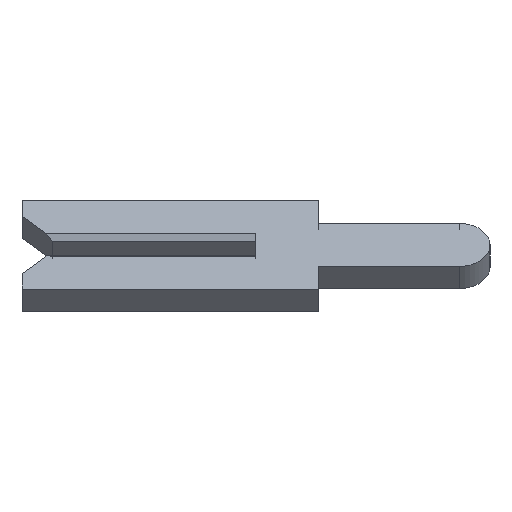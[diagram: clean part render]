
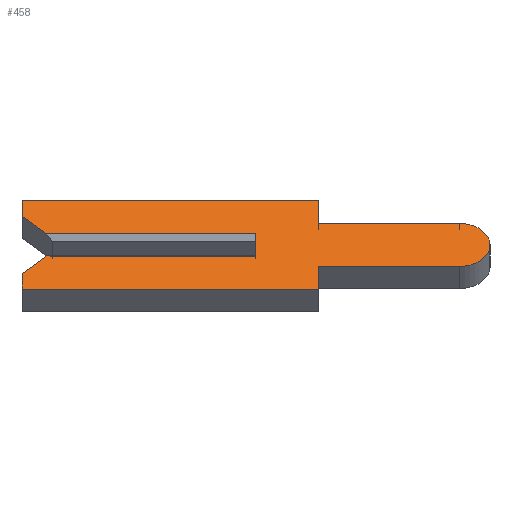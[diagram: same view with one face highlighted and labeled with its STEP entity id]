
A CAD part, left-side view. The second image highlights one B-rep face of the part: STEP entity #458.
In plain terms, the highlighted face is planar.
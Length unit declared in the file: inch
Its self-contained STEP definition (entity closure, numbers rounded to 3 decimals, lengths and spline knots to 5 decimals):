
#2 = LINE ( 'NONE', #1080, #922 ) ;
#7 = DIRECTION ( 'NONE',  ( 1., 0., 0. ) ) ;
#23 = VECTOR ( 'NONE', #225, 39.37008 ) ;
#26 = EDGE_CURVE ( 'NONE', #195, #709, #1039, .T. ) ;
#31 = CARTESIAN_POINT ( 'NONE',  ( -0.01, 0.15, -0.026 ) ) ;
#93 = DIRECTION ( 'NONE',  ( 0., 0., 1. ) ) ;
#110 = CARTESIAN_POINT ( 'NONE',  ( -0.01, -0.04, -0.0195 ) ) ;
#112 = LINE ( 'NONE', #1411, #1295 ) ;
#128 = CARTESIAN_POINT ( 'NONE',  ( -0.01, -0.1305, -0.01 ) ) ;
#134 = VERTEX_POINT ( 'NONE', #1255 ) ;
#145 = VERTEX_POINT ( 'NONE', #1369 ) ;
#151 = CARTESIAN_POINT ( 'NONE',  ( -0.01, 0.15, -0.04 ) ) ;
#164 = VECTOR ( 'NONE', #1148, 39.37008 ) ;
#171 = EDGE_CURVE ( 'NONE', #862, #134, #112, .T. ) ;
#195 = VERTEX_POINT ( 'NONE', #31 ) ;
#196 = ORIENTED_EDGE ( 'NONE', *, *, #905, .T. ) ;
#206 = CARTESIAN_POINT ( 'NONE',  ( -0.01, -0.04, 0.0195 ) ) ;
#217 = VECTOR ( 'NONE', #1092, 39.37008 ) ;
#225 = DIRECTION ( 'NONE',  ( 0., 1., 0. ) ) ;
#230 = PLANE ( 'NONE',  #634 ) ;
#232 = LINE ( 'NONE', #331, #1426 ) ;
#240 = DIRECTION ( 'NONE',  ( 0., 0., -1. ) ) ;
#322 = VECTOR ( 'NONE', #93, 39.37008 ) ;
#331 = CARTESIAN_POINT ( 'NONE',  ( -0.01, -0.04, 0.04 ) ) ;
#356 = DIRECTION ( 'NONE',  ( 0., -0.707, 0.707 ) ) ;
#371 = DIRECTION ( 'NONE',  ( 0., 0.707, 0.707 ) ) ;
#383 = VERTEX_POINT ( 'NONE', #485 ) ;
#386 = ORIENTED_EDGE ( 'NONE', *, *, #1332, .F. ) ;
#391 = EDGE_CURVE ( 'NONE', #709, #1100, #506, .T. ) ;
#402 = CARTESIAN_POINT ( 'NONE',  ( -0.01, 0.134, -0.01 ) ) ;
#404 = VERTEX_POINT ( 'NONE', #1053 ) ;
#419 = CARTESIAN_POINT ( 'NONE',  ( -0.01, 0.15, 0.04 ) ) ;
#427 = CARTESIAN_POINT ( 'NONE',  ( -0.01, 0.15, 0.026 ) ) ;
#437 = CARTESIAN_POINT ( 'NONE',  ( -0.01, -0.1305, 0. ) ) ;
#441 = DIRECTION ( 'NONE',  ( 0., 0., -1. ) ) ;
#458 = ADVANCED_FACE ( 'NONE', ( #955 ), #230, .F. ) ;
#465 = VECTOR ( 'NONE', #1323, 39.37008 ) ;
#485 = CARTESIAN_POINT ( 'NONE',  ( -0.01, -0.04, 0.04 ) ) ;
#504 = CARTESIAN_POINT ( 'NONE',  ( -0.01, -0.04, -0.04 ) ) ;
#506 = LINE ( 'NONE', #128, #164 ) ;
#536 = VECTOR ( 'NONE', #441, 39.37008 ) ;
#556 = CARTESIAN_POINT ( 'NONE',  ( -0.01, 0.15, -0.026 ) ) ;
#571 = CARTESIAN_POINT ( 'NONE',  ( -0.01, -0.1305, 0. ) ) ;
#600 = VERTEX_POINT ( 'NONE', #504 ) ;
#602 = ORIENTED_EDGE ( 'NONE', *, *, #832, .F. ) ;
#623 = CARTESIAN_POINT ( 'NONE',  ( -0.01, 0.134, 0.01 ) ) ;
#634 = AXIS2_PLACEMENT_3D ( 'NONE', #571, #7, #240 ) ;
#644 = ORIENTED_EDGE ( 'NONE', *, *, #171, .F. ) ;
#654 = DIRECTION ( 'NONE',  ( 0., 0., -1. ) ) ;
#663 = VECTOR ( 'NONE', #860, 39.37008 ) ;
#702 = VERTEX_POINT ( 'NONE', #151 ) ;
#706 = ORIENTED_EDGE ( 'NONE', *, *, #959, .F. ) ;
#709 = VERTEX_POINT ( 'NONE', #402 ) ;
#731 = CARTESIAN_POINT ( 'NONE',  ( -0.01, 0., 0.01 ) ) ;
#734 = CARTESIAN_POINT ( 'NONE',  ( -0.01, 0.15, 0.04 ) ) ;
#744 = DIRECTION ( 'NONE',  ( 0., -1., 0. ) ) ;
#755 = CARTESIAN_POINT ( 'NONE',  ( -0.01, 0., -0.01 ) ) ;
#769 = ORIENTED_EDGE ( 'NONE', *, *, #904, .F. ) ;
#773 = ORIENTED_EDGE ( 'NONE', *, *, #1248, .F. ) ;
#774 = VECTOR ( 'NONE', #744, 39.37008 ) ;
#777 = DIRECTION ( 'NONE',  ( 0., -1., 0. ) ) ;
#832 = EDGE_CURVE ( 'NONE', #1100, #943, #2, .T. ) ;
#851 = LINE ( 'NONE', #985, #465 ) ;
#852 = EDGE_CURVE ( 'NONE', #600, #702, #851, .T. ) ;
#860 = DIRECTION ( 'NONE',  ( 0., 0., 1. ) ) ;
#862 = VERTEX_POINT ( 'NONE', #623 ) ;
#866 = AXIS2_PLACEMENT_3D ( 'NONE', #437, #992, #654 ) ;
#874 = CARTESIAN_POINT ( 'NONE',  ( -0.01, -0.04, -0.0195 ) ) ;
#875 = LINE ( 'NONE', #556, #322 ) ;
#901 = VERTEX_POINT ( 'NONE', #1217 ) ;
#904 = EDGE_CURVE ( 'NONE', #134, #916, #1209, .T. ) ;
#905 = EDGE_CURVE ( 'NONE', #862, #943, #1079, .T. ) ;
#916 = VERTEX_POINT ( 'NONE', #419 ) ;
#917 = CIRCLE ( 'NONE', #866, 0.0195 ) ;
#922 = VECTOR ( 'NONE', #1099, 39.37008 ) ;
#943 = VERTEX_POINT ( 'NONE', #731 ) ;
#955 = FACE_OUTER_BOUND ( 'NONE', #1285, .T. ) ;
#959 = EDGE_CURVE ( 'NONE', #916, #383, #1350, .T. ) ;
#962 = ORIENTED_EDGE ( 'NONE', *, *, #391, .F. ) ;
#966 = CARTESIAN_POINT ( 'NONE',  ( -0.01, 0.15, 0.01 ) ) ;
#976 = LINE ( 'NONE', #1114, #536 ) ;
#985 = CARTESIAN_POINT ( 'NONE',  ( -0.01, 0.15, -0.04 ) ) ;
#992 = DIRECTION ( 'NONE',  ( 1., 0., 0. ) ) ;
#994 = EDGE_CURVE ( 'NONE', #1312, #600, #976, .T. ) ;
#1008 = DIRECTION ( 'NONE',  ( 0., 0., -1. ) ) ;
#1017 = EDGE_CURVE ( 'NONE', #404, #145, #1293, .T. ) ;
#1039 = LINE ( 'NONE', #1129, #1093 ) ;
#1053 = CARTESIAN_POINT ( 'NONE',  ( -0.01, -0.04, 0.0195 ) ) ;
#1065 = ORIENTED_EDGE ( 'NONE', *, *, #1249, .F. ) ;
#1079 = LINE ( 'NONE', #966, #774 ) ;
#1080 = CARTESIAN_POINT ( 'NONE',  ( -0.01, 0., 0.0065 ) ) ;
#1092 = DIRECTION ( 'NONE',  ( 0., -1., 0. ) ) ;
#1093 = VECTOR ( 'NONE', #356, 39.37008 ) ;
#1099 = DIRECTION ( 'NONE',  ( 0., 0., 1. ) ) ;
#1100 = VERTEX_POINT ( 'NONE', #755 ) ;
#1108 = EDGE_CURVE ( 'NONE', #702, #195, #875, .T. ) ;
#1113 = ORIENTED_EDGE ( 'NONE', *, *, #1017, .F. ) ;
#1114 = CARTESIAN_POINT ( 'NONE',  ( -0.01, -0.04, -0.04 ) ) ;
#1129 = CARTESIAN_POINT ( 'NONE',  ( -0.01, 0.1305, -0.0065 ) ) ;
#1133 = ORIENTED_EDGE ( 'NONE', *, *, #26, .F. ) ;
#1148 = DIRECTION ( 'NONE',  ( 0., -1., 0. ) ) ;
#1189 = LINE ( 'NONE', #110, #23 ) ;
#1209 = LINE ( 'NONE', #427, #663 ) ;
#1217 = CARTESIAN_POINT ( 'NONE',  ( -0.01, -0.1305, -0.0195 ) ) ;
#1248 = EDGE_CURVE ( 'NONE', #145, #901, #917, .T. ) ;
#1249 = EDGE_CURVE ( 'NONE', #383, #404, #232, .T. ) ;
#1255 = CARTESIAN_POINT ( 'NONE',  ( -0.01, 0.15, 0.026 ) ) ;
#1285 = EDGE_LOOP ( 'NONE', ( #196, #602, #962, #1133, #1326, #1384, #1311, #386, #773, #1113, #1065, #706, #769, #644 ) ) ;
#1293 = LINE ( 'NONE', #206, #1390 ) ;
#1295 = VECTOR ( 'NONE', #371, 39.37008 ) ;
#1311 = ORIENTED_EDGE ( 'NONE', *, *, #994, .F. ) ;
#1312 = VERTEX_POINT ( 'NONE', #874 ) ;
#1323 = DIRECTION ( 'NONE',  ( 0., 1., 0. ) ) ;
#1326 = ORIENTED_EDGE ( 'NONE', *, *, #1108, .F. ) ;
#1332 = EDGE_CURVE ( 'NONE', #901, #1312, #1189, .T. ) ;
#1350 = LINE ( 'NONE', #734, #217 ) ;
#1369 = CARTESIAN_POINT ( 'NONE',  ( -0.01, -0.1305, 0.0195 ) ) ;
#1384 = ORIENTED_EDGE ( 'NONE', *, *, #852, .F. ) ;
#1390 = VECTOR ( 'NONE', #777, 39.37008 ) ;
#1411 = CARTESIAN_POINT ( 'NONE',  ( -0.01, 0.1305, 0.0065 ) ) ;
#1426 = VECTOR ( 'NONE', #1008, 39.37008 ) ;
